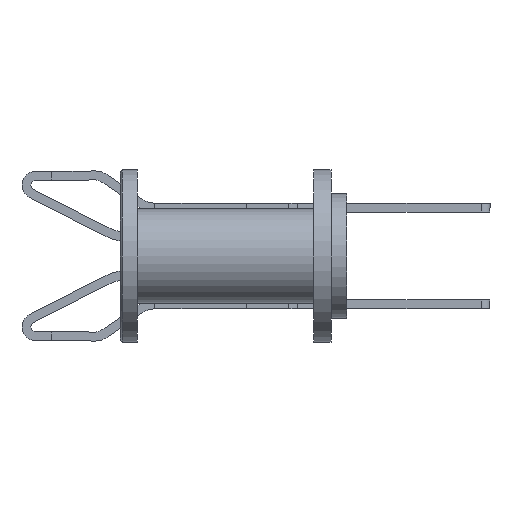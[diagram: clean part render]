
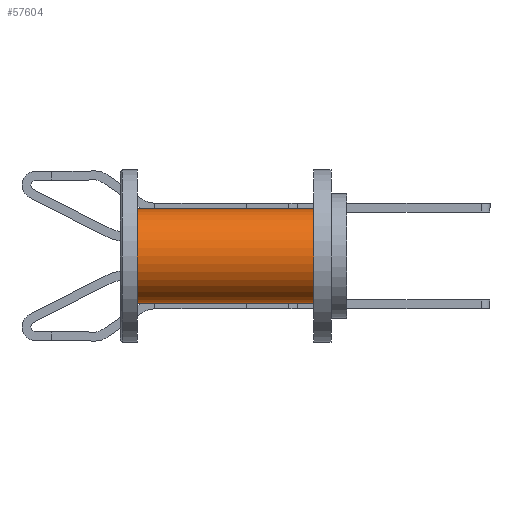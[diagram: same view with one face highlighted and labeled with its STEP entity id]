
A CAD part, left-side view. The second image highlights one B-rep face of the part: STEP entity #57604.
In plain terms, the highlighted cylindrical face has radius 1.727 mm (diameter 3.454 mm), a partial arc.
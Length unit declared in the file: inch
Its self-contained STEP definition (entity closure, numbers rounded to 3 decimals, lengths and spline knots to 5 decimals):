
#6434 = CIRCLE ( 'NONE', #48965, 0.068 ) ;
#6835 = VERTEX_POINT ( 'NONE', #15713 ) ;
#7460 = VECTOR ( 'NONE', #34223, 39.37008 ) ;
#7828 = VERTEX_POINT ( 'NONE', #49428 ) ;
#9200 = DIRECTION ( 'NONE',  ( 0., 1., 0. ) ) ;
#9808 = DIRECTION ( 'NONE',  ( 0., 1., 0. ) ) ;
#11160 = ORIENTED_EDGE ( 'NONE', *, *, #33735, .T. ) ;
#11562 = CARTESIAN_POINT ( 'NONE',  ( 0., 0.328, 0.068 ) ) ;
#12262 = CARTESIAN_POINT ( 'NONE',  ( 0., 0.025, 0.068 ) ) ;
#13222 = AXIS2_PLACEMENT_3D ( 'NONE', #36395, #9200, #40864 ) ;
#15713 = CARTESIAN_POINT ( 'NONE',  ( 0., 0.025, -0.068 ) ) ;
#16571 = EDGE_CURVE ( 'NONE', #7828, #20311, #31699, .T. ) ;
#16993 = DIRECTION ( 'NONE',  ( 0., 0., -1. ) ) ;
#17194 = ORIENTED_EDGE ( 'NONE', *, *, #16571, .T. ) ;
#20311 = VERTEX_POINT ( 'NONE', #12262 ) ;
#20708 = EDGE_LOOP ( 'NONE', ( #22415, #17194, #11160, #25416 ) ) ;
#21233 = FACE_OUTER_BOUND ( 'NONE', #20708, .T. ) ;
#22415 = ORIENTED_EDGE ( 'NONE', *, *, #27930, .F. ) ;
#22664 = CARTESIAN_POINT ( 'NONE',  ( 0., 0.28, -0.068 ) ) ;
#25416 = ORIENTED_EDGE ( 'NONE', *, *, #26417, .F. ) ;
#26417 = EDGE_CURVE ( 'NONE', #53281, #6835, #41067, .T. ) ;
#27930 = EDGE_CURVE ( 'NONE', #7828, #53281, #41572, .T. ) ;
#30516 = DIRECTION ( 'NONE',  ( 0., -1., 0. ) ) ;
#30644 = VECTOR ( 'NONE', #53382, 39.37008 ) ;
#31699 = LINE ( 'NONE', #11562, #7460 ) ;
#33735 = EDGE_CURVE ( 'NONE', #20311, #6835, #6434, .T. ) ;
#34223 = DIRECTION ( 'NONE',  ( 0., -1., 0. ) ) ;
#36395 = CARTESIAN_POINT ( 'NONE',  ( 0., 0.28, 0. ) ) ;
#36966 = CARTESIAN_POINT ( 'NONE',  ( 0., 0.025, 0. ) ) ;
#39953 = CARTESIAN_POINT ( 'NONE',  ( 0., 0.328, -0.068 ) ) ;
#40864 = DIRECTION ( 'NONE',  ( 0., 0., 1. ) ) ;
#41067 = LINE ( 'NONE', #39953, #30644 ) ;
#41437 = DIRECTION ( 'NONE',  ( 0., 0., 1. ) ) ;
#41572 = CIRCLE ( 'NONE', #13222, 0.068 ) ;
#43941 = CARTESIAN_POINT ( 'NONE',  ( 0., 0.328, 0. ) ) ;
#45227 = AXIS2_PLACEMENT_3D ( 'NONE', #43941, #30516, #16993 ) ;
#48965 = AXIS2_PLACEMENT_3D ( 'NONE', #36966, #9808, #41437 ) ;
#49428 = CARTESIAN_POINT ( 'NONE',  ( 0., 0.28, 0.068 ) ) ;
#53281 = VERTEX_POINT ( 'NONE', #22664 ) ;
#53382 = DIRECTION ( 'NONE',  ( 0., -1., 0. ) ) ;
#55521 = CYLINDRICAL_SURFACE ( 'NONE', #45227, 0.068 ) ;
#57604 = ADVANCED_FACE ( 'NONE', ( #21233 ), #55521, .T. ) ;
